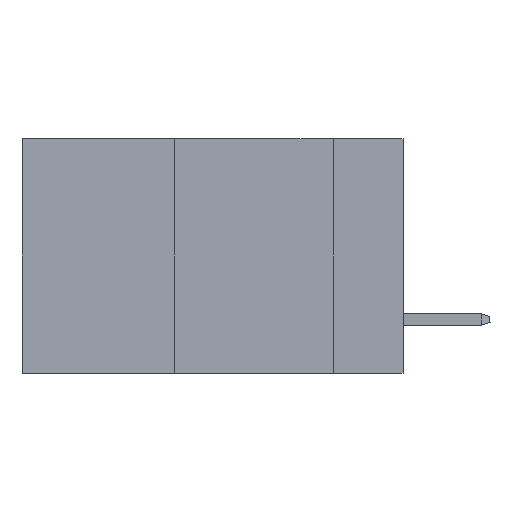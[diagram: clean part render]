
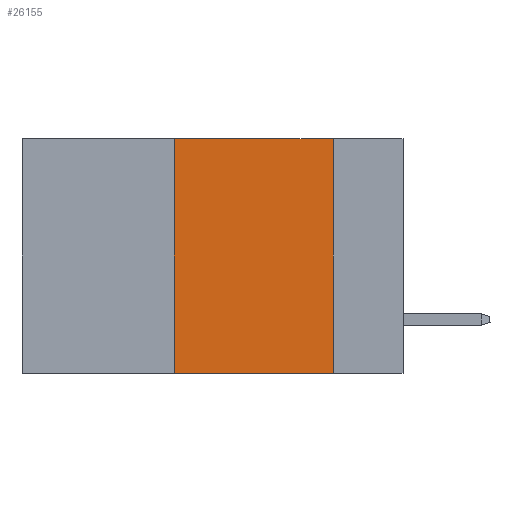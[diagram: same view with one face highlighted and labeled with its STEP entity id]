
A CAD part, left-side view. The second image highlights one B-rep face of the part: STEP entity #26155.
In plain terms, the highlighted planar face has unit normal (-1, 0, 0).
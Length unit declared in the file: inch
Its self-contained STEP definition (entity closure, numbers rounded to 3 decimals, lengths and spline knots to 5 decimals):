
#173 = CARTESIAN_POINT ( 'NONE',  ( 0., 0.36, 0. ) ) ;
#708 = CARTESIAN_POINT ( 'NONE',  ( 0., 0.11, -0.37 ) ) ;
#2574 = DIRECTION ( 'NONE',  ( 0., 0., -1. ) ) ;
#4061 = CARTESIAN_POINT ( 'NONE',  ( 0., 0.6, 0. ) ) ;
#5874 = LINE ( 'NONE', #19338, #20633 ) ;
#6442 = CARTESIAN_POINT ( 'NONE',  ( 0., 0.6, -0.37 ) ) ;
#7112 = VECTOR ( 'NONE', #26549, 39.37008 ) ;
#7863 = CARTESIAN_POINT ( 'NONE',  ( 0., 0.6, 0. ) ) ;
#8029 = VERTEX_POINT ( 'NONE', #42248 ) ;
#9251 = AXIS2_PLACEMENT_3D ( 'NONE', #4061, #17513, #20402 ) ;
#9438 = VECTOR ( 'NONE', #13840, 39.37008 ) ;
#10723 = CARTESIAN_POINT ( 'NONE',  ( 0., 0.36, -0.37 ) ) ;
#12300 = ORIENTED_EDGE ( 'NONE', *, *, #27291, .F. ) ;
#13840 = DIRECTION ( 'NONE',  ( 0., 0., 1. ) ) ;
#14495 = LINE ( 'NONE', #7863, #23561 ) ;
#17513 = DIRECTION ( 'NONE',  ( 1., 0., 0. ) ) ;
#18442 = EDGE_LOOP ( 'NONE', ( #12300, #39940, #40194, #29690 ) ) ;
#19338 = CARTESIAN_POINT ( 'NONE',  ( 0., 0.11, 0. ) ) ;
#20402 = DIRECTION ( 'NONE',  ( 0., 0., -1. ) ) ;
#20633 = VECTOR ( 'NONE', #2574, 39.37008 ) ;
#22730 = VERTEX_POINT ( 'NONE', #708 ) ;
#23502 = CARTESIAN_POINT ( 'NONE',  ( 0., 0.36, 0. ) ) ;
#23561 = VECTOR ( 'NONE', #27521, 39.37008 ) ;
#23864 = LINE ( 'NONE', #6442, #7112 ) ;
#25740 = VERTEX_POINT ( 'NONE', #10723 ) ;
#26155 = ADVANCED_FACE ( 'NONE', ( #37787 ), #37563, .F. ) ;
#26549 = DIRECTION ( 'NONE',  ( 0., -1., 0. ) ) ;
#27291 = EDGE_CURVE ( 'NONE', #8029, #22730, #5874, .T. ) ;
#27521 = DIRECTION ( 'NONE',  ( 0., -1., 0. ) ) ;
#29690 = ORIENTED_EDGE ( 'NONE', *, *, #41866, .T. ) ;
#30053 = VERTEX_POINT ( 'NONE', #23502 ) ;
#30840 = EDGE_CURVE ( 'NONE', #30053, #8029, #14495, .T. ) ;
#30852 = EDGE_CURVE ( 'NONE', #25740, #30053, #34767, .T. ) ;
#34767 = LINE ( 'NONE', #173, #9438 ) ;
#37563 = PLANE ( 'NONE',  #9251 ) ;
#37787 = FACE_OUTER_BOUND ( 'NONE', #18442, .T. ) ;
#39940 = ORIENTED_EDGE ( 'NONE', *, *, #30840, .F. ) ;
#40194 = ORIENTED_EDGE ( 'NONE', *, *, #30852, .F. ) ;
#41866 = EDGE_CURVE ( 'NONE', #25740, #22730, #23864, .T. ) ;
#42248 = CARTESIAN_POINT ( 'NONE',  ( 0., 0.11, 0. ) ) ;
